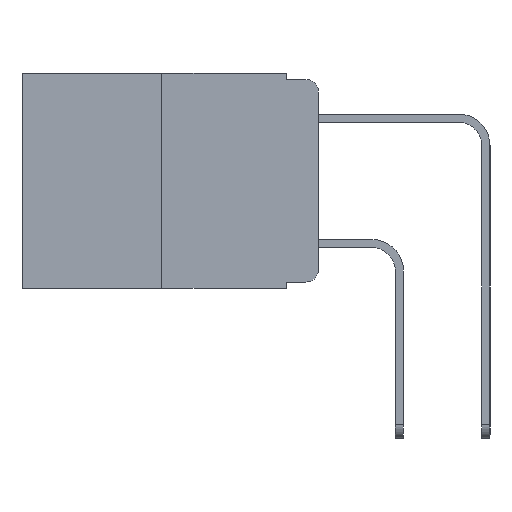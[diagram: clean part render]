
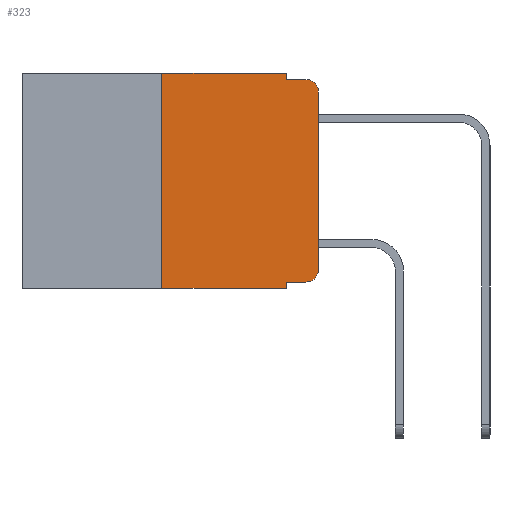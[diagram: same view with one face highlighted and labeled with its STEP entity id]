
A CAD part, left-side view. The second image highlights one B-rep face of the part: STEP entity #323.
In plain terms, the highlighted planar face has unit normal (-1, 0, 0).
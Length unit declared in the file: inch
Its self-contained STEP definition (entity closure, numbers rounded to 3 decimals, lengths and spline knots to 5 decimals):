
#263 = DIRECTION ( 'NONE',  ( 0., -1., 0. ) ) ;
#323 = ADVANCED_FACE ( 'NONE', ( #11592 ), #7920, .F. ) ;
#392 = ORIENTED_EDGE ( 'NONE', *, *, #3526, .T. ) ;
#407 = ORIENTED_EDGE ( 'NONE', *, *, #2890, .F. ) ;
#713 = CARTESIAN_POINT ( 'NONE',  ( 0., 0., -0.313 ) ) ;
#775 = LINE ( 'NONE', #1266, #10201 ) ;
#887 = ORIENTED_EDGE ( 'NONE', *, *, #2208, .F. ) ;
#1084 = VECTOR ( 'NONE', #263, 39.37008 ) ;
#1171 = DIRECTION ( 'NONE',  ( 0., 0., 1. ) ) ;
#1181 = ORIENTED_EDGE ( 'NONE', *, *, #4208, .T. ) ;
#1226 = CARTESIAN_POINT ( 'NONE',  ( 0., 0.051, -0.01 ) ) ;
#1257 = VERTEX_POINT ( 'NONE', #6284 ) ;
#1266 = CARTESIAN_POINT ( 'NONE',  ( 0., 0.25, 0. ) ) ;
#1433 = ORIENTED_EDGE ( 'NONE', *, *, #10769, .T. ) ;
#1502 = EDGE_CURVE ( 'NONE', #3646, #1907, #775, .T. ) ;
#1534 = CARTESIAN_POINT ( 'NONE',  ( 0., 0.051, 0. ) ) ;
#1728 = EDGE_LOOP ( 'NONE', ( #1181, #392, #407, #887, #6208, #2836, #2549, #2741, #1433, #6160 ) ) ;
#1744 = DIRECTION ( 'NONE',  ( -1., 0., 0. ) ) ;
#1869 = VECTOR ( 'NONE', #7924, 39.37008 ) ;
#1907 = VERTEX_POINT ( 'NONE', #6210 ) ;
#2075 = CARTESIAN_POINT ( 'NONE',  ( 0., 0.051, 0. ) ) ;
#2156 = CARTESIAN_POINT ( 'NONE',  ( 0., 0.051, -0.01 ) ) ;
#2165 = CARTESIAN_POINT ( 'NONE',  ( 0., 0.02, -0.01 ) ) ;
#2208 = EDGE_CURVE ( 'NONE', #5917, #9913, #9012, .T. ) ;
#2549 = ORIENTED_EDGE ( 'NONE', *, *, #9290, .T. ) ;
#2607 = DIRECTION ( 'NONE',  ( 0., -1., 0. ) ) ;
#2741 = ORIENTED_EDGE ( 'NONE', *, *, #11307, .F. ) ;
#2836 = ORIENTED_EDGE ( 'NONE', *, *, #1502, .F. ) ;
#2890 = EDGE_CURVE ( 'NONE', #9913, #3993, #8687, .T. ) ;
#3247 = CARTESIAN_POINT ( 'NONE',  ( 0., 0., -0.03 ) ) ;
#3317 = VECTOR ( 'NONE', #2607, 39.37008 ) ;
#3526 = EDGE_CURVE ( 'NONE', #9975, #3993, #9053, .T. ) ;
#3646 = VERTEX_POINT ( 'NONE', #9888 ) ;
#3855 = DIRECTION ( 'NONE',  ( 1., 0., 0. ) ) ;
#3993 = VERTEX_POINT ( 'NONE', #2165 ) ;
#4148 = CARTESIAN_POINT ( 'NONE',  ( 0., 0.051, 0. ) ) ;
#4208 = EDGE_CURVE ( 'NONE', #10243, #9975, #4759, .T. ) ;
#4218 = DIRECTION ( 'NONE',  ( 0., 0., -1. ) ) ;
#4297 = LINE ( 'NONE', #4148, #6351 ) ;
#4344 = CARTESIAN_POINT ( 'NONE',  ( 0., 0.051, -0.333 ) ) ;
#4630 = AXIS2_PLACEMENT_3D ( 'NONE', #7944, #3855, #4218 ) ;
#4759 = LINE ( 'NONE', #8676, #1869 ) ;
#5017 = AXIS2_PLACEMENT_3D ( 'NONE', #7310, #1744, #8237 ) ;
#5043 = VECTOR ( 'NONE', #7716, 39.37008 ) ;
#5094 = VERTEX_POINT ( 'NONE', #8115 ) ;
#5702 = VECTOR ( 'NONE', #10405, 39.37008 ) ;
#5917 = VERTEX_POINT ( 'NONE', #2075 ) ;
#6002 = CARTESIAN_POINT ( 'NONE',  ( 0., 0.473, -0.343 ) ) ;
#6160 = ORIENTED_EDGE ( 'NONE', *, *, #10258, .T. ) ;
#6208 = ORIENTED_EDGE ( 'NONE', *, *, #7723, .F. ) ;
#6210 = CARTESIAN_POINT ( 'NONE',  ( 0., 0.25, 0. ) ) ;
#6284 = CARTESIAN_POINT ( 'NONE',  ( 0., 0.051, -0.333 ) ) ;
#6351 = VECTOR ( 'NONE', #7684, 39.37008 ) ;
#7310 = CARTESIAN_POINT ( 'NONE',  ( 0., 0.02, -0.313 ) ) ;
#7375 = LINE ( 'NONE', #7783, #5043 ) ;
#7684 = DIRECTION ( 'NONE',  ( 0., 0., -1. ) ) ;
#7716 = DIRECTION ( 'NONE',  ( 0., -1., 0. ) ) ;
#7723 = EDGE_CURVE ( 'NONE', #1907, #5917, #7375, .T. ) ;
#7783 = CARTESIAN_POINT ( 'NONE',  ( 0., 0.473, 0. ) ) ;
#7920 = PLANE ( 'NONE',  #4630 ) ;
#7924 = DIRECTION ( 'NONE',  ( 0., 0., 1. ) ) ;
#7944 = CARTESIAN_POINT ( 'NONE',  ( 0., 0.473, 0. ) ) ;
#8115 = CARTESIAN_POINT ( 'NONE',  ( 0., 0.051, -0.343 ) ) ;
#8237 = DIRECTION ( 'NONE',  ( 0., 0., -1. ) ) ;
#8268 = DIRECTION ( 'NONE',  ( 0., 0., -1. ) ) ;
#8676 = CARTESIAN_POINT ( 'NONE',  ( 0., 0., 0. ) ) ;
#8687 = LINE ( 'NONE', #1226, #3317 ) ;
#9012 = LINE ( 'NONE', #1534, #11161 ) ;
#9053 = CIRCLE ( 'NONE', #9597, 0.02 ) ;
#9133 = CIRCLE ( 'NONE', #5017, 0.02 ) ;
#9290 = EDGE_CURVE ( 'NONE', #3646, #5094, #10202, .T. ) ;
#9597 = AXIS2_PLACEMENT_3D ( 'NONE', #10005, #9983, #9981 ) ;
#9777 = LINE ( 'NONE', #4344, #5702 ) ;
#9888 = CARTESIAN_POINT ( 'NONE',  ( 0., 0.25, -0.343 ) ) ;
#9913 = VERTEX_POINT ( 'NONE', #2156 ) ;
#9975 = VERTEX_POINT ( 'NONE', #3247 ) ;
#9981 = DIRECTION ( 'NONE',  ( 0., 0., -1. ) ) ;
#9983 = DIRECTION ( 'NONE',  ( -1., 0., 0. ) ) ;
#10005 = CARTESIAN_POINT ( 'NONE',  ( 0., 0.02, -0.03 ) ) ;
#10063 = CARTESIAN_POINT ( 'NONE',  ( 0., 0.02, -0.333 ) ) ;
#10201 = VECTOR ( 'NONE', #1171, 39.37008 ) ;
#10202 = LINE ( 'NONE', #6002, #1084 ) ;
#10243 = VERTEX_POINT ( 'NONE', #713 ) ;
#10258 = EDGE_CURVE ( 'NONE', #10370, #10243, #9133, .T. ) ;
#10370 = VERTEX_POINT ( 'NONE', #10063 ) ;
#10405 = DIRECTION ( 'NONE',  ( 0., -1., 0. ) ) ;
#10769 = EDGE_CURVE ( 'NONE', #1257, #10370, #9777, .T. ) ;
#11161 = VECTOR ( 'NONE', #8268, 39.37008 ) ;
#11307 = EDGE_CURVE ( 'NONE', #1257, #5094, #4297, .T. ) ;
#11592 = FACE_OUTER_BOUND ( 'NONE', #1728, .T. ) ;
